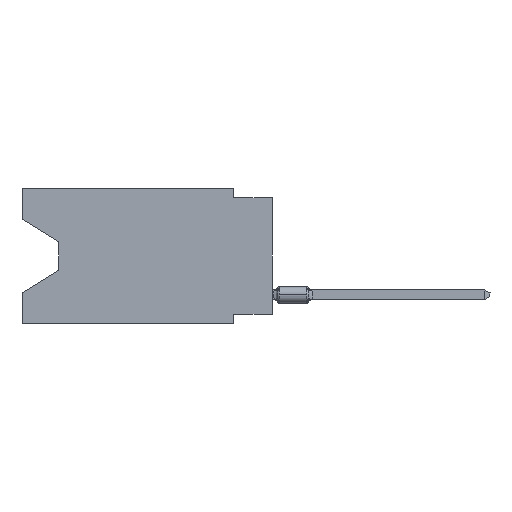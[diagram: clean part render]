
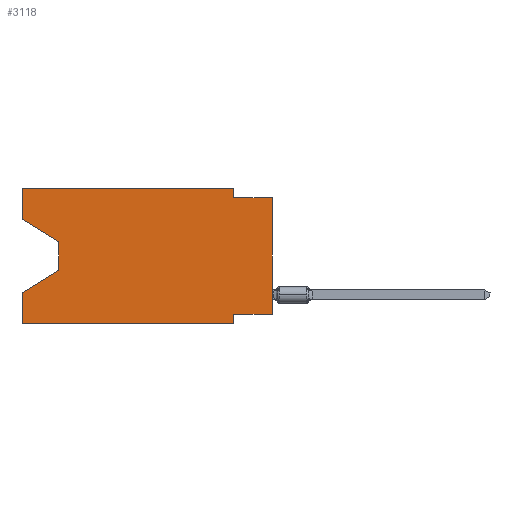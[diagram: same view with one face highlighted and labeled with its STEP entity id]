
A CAD part, left-side view. The second image highlights one B-rep face of the part: STEP entity #3118.
In plain terms, the highlighted planar face has unit normal (-1, 0, 0).
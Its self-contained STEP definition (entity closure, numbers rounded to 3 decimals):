
#206 = ORIENTED_EDGE ( 'NONE', *, *, #22914, .T. ) ;
#509 = CARTESIAN_POINT ( 'NONE',  ( 0., 2.54, -8.255 ) ) ;
#1017 = CARTESIAN_POINT ( 'NONE',  ( 0., 16.383, 0. ) ) ;
#1356 = ORIENTED_EDGE ( 'NONE', *, *, #21935, .T. ) ;
#2915 = VERTEX_POINT ( 'NONE', #25843 ) ;
#3000 = CARTESIAN_POINT ( 'NONE',  ( 0., 2.54, 0. ) ) ;
#3118 = ADVANCED_FACE ( 'NONE', ( #18323 ), #7021, .F. ) ;
#3186 = EDGE_CURVE ( 'NONE', #29886, #34936, #15942, .T. ) ;
#4054 = ORIENTED_EDGE ( 'NONE', *, *, #22308, .F. ) ;
#4058 = DIRECTION ( 'NONE',  ( 0., 1., 0. ) ) ;
#4468 = DIRECTION ( 'NONE',  ( 0., 0., -1. ) ) ;
#4482 = LINE ( 'NONE', #26745, #10454 ) ;
#4553 = LINE ( 'NONE', #26987, #34966 ) ;
#5477 = DIRECTION ( 'NONE',  ( 0., 0., 1. ) ) ;
#6542 = VECTOR ( 'NONE', #9989, 1000. ) ;
#7021 = PLANE ( 'NONE',  #15172 ) ;
#7210 = EDGE_CURVE ( 'NONE', #18366, #2915, #31299, .T. ) ;
#7358 = VERTEX_POINT ( 'NONE', #29268 ) ;
#7599 = LINE ( 'NONE', #22023, #25066 ) ;
#8066 = CARTESIAN_POINT ( 'NONE',  ( 0., 0., -8.255 ) ) ;
#8371 = VERTEX_POINT ( 'NONE', #509 ) ;
#8495 = EDGE_CURVE ( 'NONE', #8371, #32494, #17830, .T. ) ;
#9115 = VECTOR ( 'NONE', #17283, 1000. ) ;
#9791 = VECTOR ( 'NONE', #34045, 1000. ) ;
#9989 = DIRECTION ( 'NONE',  ( 0., 0.855, -0.519 ) ) ;
#10361 = LINE ( 'NONE', #32622, #6542 ) ;
#10454 = VECTOR ( 'NONE', #12331, 1000. ) ;
#10462 = CARTESIAN_POINT ( 'NONE',  ( 0., 2.54, -8.89 ) ) ;
#11217 = CARTESIAN_POINT ( 'NONE',  ( 0., 16.383, 0. ) ) ;
#11404 = LINE ( 'NONE', #11217, #29185 ) ;
#11434 = LINE ( 'NONE', #20188, #9791 ) ;
#11756 = DIRECTION ( 'NONE',  ( 0., 0., -1. ) ) ;
#12265 = CARTESIAN_POINT ( 'NONE',  ( 0., 2.54, -0.635 ) ) ;
#12291 = DIRECTION ( 'NONE',  ( 0., -1., 0. ) ) ;
#12331 = DIRECTION ( 'NONE',  ( 0., 0., -1. ) ) ;
#12579 = VERTEX_POINT ( 'NONE', #3000 ) ;
#12994 = ORIENTED_EDGE ( 'NONE', *, *, #33007, .F. ) ;
#14028 = ORIENTED_EDGE ( 'NONE', *, *, #20276, .F. ) ;
#14374 = VECTOR ( 'NONE', #5477, 1000. ) ;
#14744 = VERTEX_POINT ( 'NONE', #12265 ) ;
#14995 = EDGE_LOOP ( 'NONE', ( #1356, #20453, #206, #19433, #20122, #31893, #14028, #29935, #33436, #21091, #4054, #12994 ) ) ;
#15172 = AXIS2_PLACEMENT_3D ( 'NONE', #18149, #35282, #4468 ) ;
#15475 = VECTOR ( 'NONE', #11756, 1000. ) ;
#15942 = LINE ( 'NONE', #32558, #17575 ) ;
#16702 = DIRECTION ( 'NONE',  ( 0., -1., 0. ) ) ;
#17283 = DIRECTION ( 'NONE',  ( 0., 0., -1. ) ) ;
#17575 = VECTOR ( 'NONE', #26897, 1000. ) ;
#17830 = LINE ( 'NONE', #34769, #9115 ) ;
#18149 = CARTESIAN_POINT ( 'NONE',  ( 0., 16.383, 0. ) ) ;
#18207 = CARTESIAN_POINT ( 'NONE',  ( 0., 13.97, -3.505 ) ) ;
#18323 = FACE_OUTER_BOUND ( 'NONE', #14995, .T. ) ;
#18366 = VERTEX_POINT ( 'NONE', #18207 ) ;
#19433 = ORIENTED_EDGE ( 'NONE', *, *, #34993, .F. ) ;
#20122 = ORIENTED_EDGE ( 'NONE', *, *, #32444, .T. ) ;
#20188 = CARTESIAN_POINT ( 'NONE',  ( 0., 16.383, 0. ) ) ;
#20276 = EDGE_CURVE ( 'NONE', #29886, #8371, #20645, .T. ) ;
#20453 = ORIENTED_EDGE ( 'NONE', *, *, #7210, .T. ) ;
#20645 = LINE ( 'NONE', #31782, #30986 ) ;
#21091 = ORIENTED_EDGE ( 'NONE', *, *, #35146, .F. ) ;
#21290 = EDGE_CURVE ( 'NONE', #14744, #34936, #7599, .T. ) ;
#21335 = DIRECTION ( 'NONE',  ( 0., -0.855, -0.519 ) ) ;
#21935 = EDGE_CURVE ( 'NONE', #7358, #18366, #4553, .T. ) ;
#22023 = CARTESIAN_POINT ( 'NONE',  ( 0., 0., -0.635 ) ) ;
#22308 = EDGE_CURVE ( 'NONE', #28025, #12579, #11404, .T. ) ;
#22519 = VECTOR ( 'NONE', #12291, 1000. ) ;
#22882 = CARTESIAN_POINT ( 'NONE',  ( 0., 16.383, -8.89 ) ) ;
#22914 = EDGE_CURVE ( 'NONE', #2915, #35104, #10361, .T. ) ;
#25066 = VECTOR ( 'NONE', #33149, 1000. ) ;
#25459 = CARTESIAN_POINT ( 'NONE',  ( 0., 13.97, -3.505 ) ) ;
#25843 = CARTESIAN_POINT ( 'NONE',  ( 0., 13.97, -5.385 ) ) ;
#26745 = CARTESIAN_POINT ( 'NONE',  ( 0., 2.54, 0. ) ) ;
#26897 = DIRECTION ( 'NONE',  ( 0., 0., 1. ) ) ;
#26920 = CARTESIAN_POINT ( 'NONE',  ( 0., 16.383, -6.852 ) ) ;
#26987 = CARTESIAN_POINT ( 'NONE',  ( 0., 16.383, -2.038 ) ) ;
#27383 = LINE ( 'NONE', #33377, #14374 ) ;
#28025 = VERTEX_POINT ( 'NONE', #1017 ) ;
#29185 = VECTOR ( 'NONE', #16702, 1000. ) ;
#29268 = CARTESIAN_POINT ( 'NONE',  ( 0., 16.383, -2.038 ) ) ;
#29594 = VERTEX_POINT ( 'NONE', #22882 ) ;
#29886 = VERTEX_POINT ( 'NONE', #8066 ) ;
#29935 = ORIENTED_EDGE ( 'NONE', *, *, #3186, .T. ) ;
#30986 = VECTOR ( 'NONE', #4058, 1000. ) ;
#31299 = LINE ( 'NONE', #25459, #15475 ) ;
#31683 = CARTESIAN_POINT ( 'NONE',  ( 0., 0., -0.635 ) ) ;
#31782 = CARTESIAN_POINT ( 'NONE',  ( 0., 0., -8.255 ) ) ;
#31893 = ORIENTED_EDGE ( 'NONE', *, *, #8495, .F. ) ;
#32002 = LINE ( 'NONE', #34190, #22519 ) ;
#32444 = EDGE_CURVE ( 'NONE', #29594, #32494, #32002, .T. ) ;
#32494 = VERTEX_POINT ( 'NONE', #10462 ) ;
#32558 = CARTESIAN_POINT ( 'NONE',  ( 0., 0., 0. ) ) ;
#32622 = CARTESIAN_POINT ( 'NONE',  ( 0., 13.97, -5.385 ) ) ;
#33007 = EDGE_CURVE ( 'NONE', #7358, #28025, #27383, .T. ) ;
#33149 = DIRECTION ( 'NONE',  ( 0., -1., 0. ) ) ;
#33377 = CARTESIAN_POINT ( 'NONE',  ( 0., 16.383, 0. ) ) ;
#33436 = ORIENTED_EDGE ( 'NONE', *, *, #21290, .F. ) ;
#34045 = DIRECTION ( 'NONE',  ( 0., 0., 1. ) ) ;
#34190 = CARTESIAN_POINT ( 'NONE',  ( 0., 16.383, -8.89 ) ) ;
#34769 = CARTESIAN_POINT ( 'NONE',  ( 0., 2.54, -8.89 ) ) ;
#34936 = VERTEX_POINT ( 'NONE', #31683 ) ;
#34966 = VECTOR ( 'NONE', #21335, 1000. ) ;
#34993 = EDGE_CURVE ( 'NONE', #29594, #35104, #11434, .T. ) ;
#35104 = VERTEX_POINT ( 'NONE', #26920 ) ;
#35146 = EDGE_CURVE ( 'NONE', #12579, #14744, #4482, .T. ) ;
#35282 = DIRECTION ( 'NONE',  ( 1., 0., 0. ) ) ;
